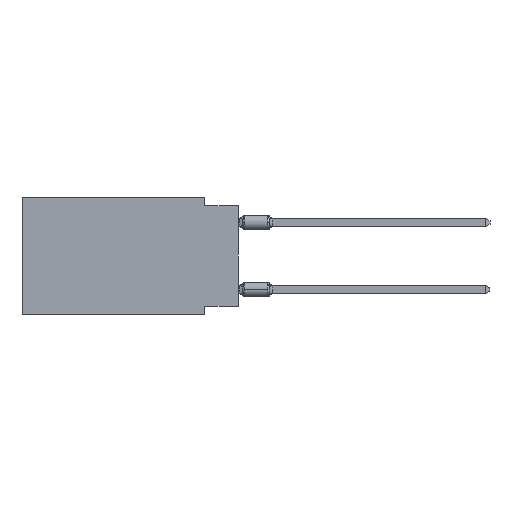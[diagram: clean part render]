
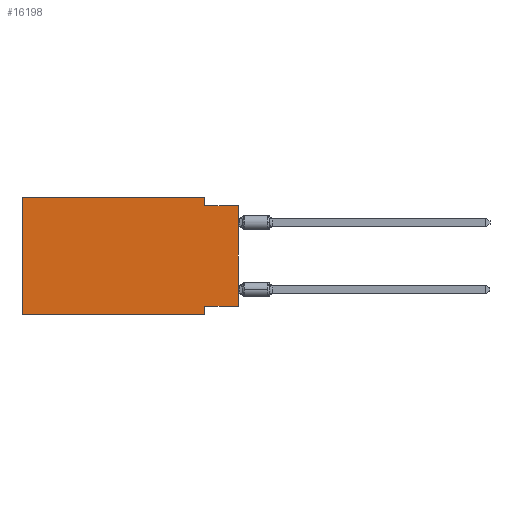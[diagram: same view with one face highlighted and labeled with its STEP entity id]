
A CAD part, left-side view. The second image highlights one B-rep face of the part: STEP entity #16198.
In plain terms, the highlighted planar face has unit normal (-1, 0, 0).
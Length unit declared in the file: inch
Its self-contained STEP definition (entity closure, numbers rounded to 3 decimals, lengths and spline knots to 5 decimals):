
#507 = CARTESIAN_POINT ( 'NONE',  ( 0., 0., -0.325 ) ) ;
#1373 = VECTOR ( 'NONE', #16135, 39.37008 ) ;
#1617 = CARTESIAN_POINT ( 'NONE',  ( 0., 0., -0.025 ) ) ;
#2565 = ORIENTED_EDGE ( 'NONE', *, *, #13307, .F. ) ;
#2780 = ORIENTED_EDGE ( 'NONE', *, *, #19507, .F. ) ;
#2788 = CARTESIAN_POINT ( 'NONE',  ( 0., 0.1, 0. ) ) ;
#3064 = CARTESIAN_POINT ( 'NONE',  ( 0., 0.1, -0.35 ) ) ;
#3261 = LINE ( 'NONE', #3064, #5551 ) ;
#3516 = DIRECTION ( 'NONE',  ( 0., 1., 0. ) ) ;
#4404 = CARTESIAN_POINT ( 'NONE',  ( 0., 0.645, 0. ) ) ;
#4417 = CARTESIAN_POINT ( 'NONE',  ( 0., 0., 0. ) ) ;
#4781 = VECTOR ( 'NONE', #3516, 39.37008 ) ;
#5317 = VERTEX_POINT ( 'NONE', #6682 ) ;
#5551 = VECTOR ( 'NONE', #9144, 39.37008 ) ;
#5581 = CARTESIAN_POINT ( 'NONE',  ( 0., 0.645, -0.35 ) ) ;
#5618 = VERTEX_POINT ( 'NONE', #1617 ) ;
#5624 = LINE ( 'NONE', #19045, #1373 ) ;
#5643 = ORIENTED_EDGE ( 'NONE', *, *, #10858, .F. ) ;
#5847 = DIRECTION ( 'NONE',  ( 0., 0., -1. ) ) ;
#5936 = DIRECTION ( 'NONE',  ( 1., 0., 0. ) ) ;
#5951 = CARTESIAN_POINT ( 'NONE',  ( 0., 0.645, 0. ) ) ;
#6211 = VERTEX_POINT ( 'NONE', #16164 ) ;
#6272 = LINE ( 'NONE', #507, #4781 ) ;
#6588 = VECTOR ( 'NONE', #5847, 39.37008 ) ;
#6682 = CARTESIAN_POINT ( 'NONE',  ( 0., 0.1, -0.35 ) ) ;
#7250 = FACE_OUTER_BOUND ( 'NONE', #13541, .T. ) ;
#8084 = CARTESIAN_POINT ( 'NONE',  ( 0., 0.645, 0. ) ) ;
#8522 = ORIENTED_EDGE ( 'NONE', *, *, #11735, .F. ) ;
#9144 = DIRECTION ( 'NONE',  ( 0., 0., -1. ) ) ;
#9172 = VECTOR ( 'NONE', #19459, 39.37008 ) ;
#10022 = EDGE_CURVE ( 'NONE', #17816, #5317, #5624, .T. ) ;
#10158 = CARTESIAN_POINT ( 'NONE',  ( 0., 0.1, 0. ) ) ;
#10213 = EDGE_CURVE ( 'NONE', #10215, #5618, #10770, .T. ) ;
#10215 = VERTEX_POINT ( 'NONE', #16519 ) ;
#10578 = PLANE ( 'NONE',  #11113 ) ;
#10770 = LINE ( 'NONE', #12279, #18486 ) ;
#10858 = EDGE_CURVE ( 'NONE', #6211, #18511, #17037, .T. ) ;
#11027 = ORIENTED_EDGE ( 'NONE', *, *, #11741, .T. ) ;
#11113 = AXIS2_PLACEMENT_3D ( 'NONE', #4404, #5936, #16737 ) ;
#11735 = EDGE_CURVE ( 'NONE', #18511, #10215, #14740, .T. ) ;
#11741 = EDGE_CURVE ( 'NONE', #15753, #5618, #16355, .T. ) ;
#11970 = ORIENTED_EDGE ( 'NONE', *, *, #10213, .F. ) ;
#12279 = CARTESIAN_POINT ( 'NONE',  ( 0., 0., -0.025 ) ) ;
#12309 = EDGE_CURVE ( 'NONE', #15534, #5317, #3261, .T. ) ;
#13307 = EDGE_CURVE ( 'NONE', #15753, #15534, #6272, .T. ) ;
#13541 = EDGE_LOOP ( 'NONE', ( #11027, #11970, #8522, #5643, #2780, #14969, #18382, #2565 ) ) ;
#13671 = VECTOR ( 'NONE', #16650, 39.37008 ) ;
#14652 = DIRECTION ( 'NONE',  ( 0., 0., 1. ) ) ;
#14740 = LINE ( 'NONE', #2788, #6588 ) ;
#14969 = ORIENTED_EDGE ( 'NONE', *, *, #10022, .T. ) ;
#14981 = CARTESIAN_POINT ( 'NONE',  ( 0., 0., -0.325 ) ) ;
#15534 = VERTEX_POINT ( 'NONE', #17704 ) ;
#15753 = VERTEX_POINT ( 'NONE', #14981 ) ;
#16135 = DIRECTION ( 'NONE',  ( 0., -1., 0. ) ) ;
#16164 = CARTESIAN_POINT ( 'NONE',  ( 0., 0.645, 0. ) ) ;
#16198 = ADVANCED_FACE ( 'NONE', ( #7250 ), #10578, .F. ) ;
#16262 = LINE ( 'NONE', #8084, #19869 ) ;
#16355 = LINE ( 'NONE', #4417, #9172 ) ;
#16519 = CARTESIAN_POINT ( 'NONE',  ( 0., 0.1, -0.025 ) ) ;
#16650 = DIRECTION ( 'NONE',  ( 0., -1., 0. ) ) ;
#16737 = DIRECTION ( 'NONE',  ( 0., 0., -1. ) ) ;
#17037 = LINE ( 'NONE', #5951, #13671 ) ;
#17704 = CARTESIAN_POINT ( 'NONE',  ( 0., 0.1, -0.325 ) ) ;
#17816 = VERTEX_POINT ( 'NONE', #5581 ) ;
#18026 = DIRECTION ( 'NONE',  ( 0., -1., 0. ) ) ;
#18382 = ORIENTED_EDGE ( 'NONE', *, *, #12309, .F. ) ;
#18486 = VECTOR ( 'NONE', #18026, 39.37008 ) ;
#18511 = VERTEX_POINT ( 'NONE', #10158 ) ;
#19045 = CARTESIAN_POINT ( 'NONE',  ( 0., 0.645, -0.35 ) ) ;
#19459 = DIRECTION ( 'NONE',  ( 0., 0., 1. ) ) ;
#19507 = EDGE_CURVE ( 'NONE', #17816, #6211, #16262, .T. ) ;
#19869 = VECTOR ( 'NONE', #14652, 39.37008 ) ;
